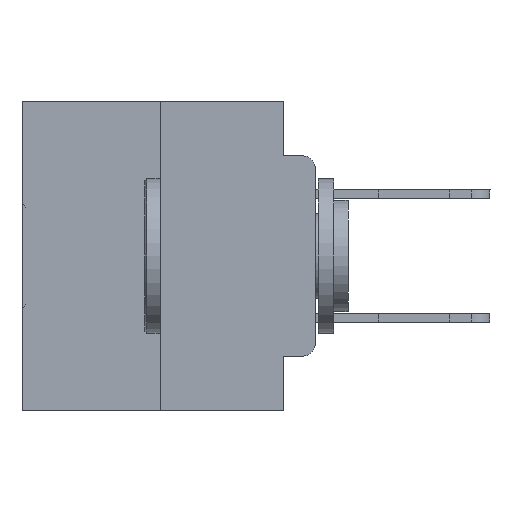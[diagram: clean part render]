
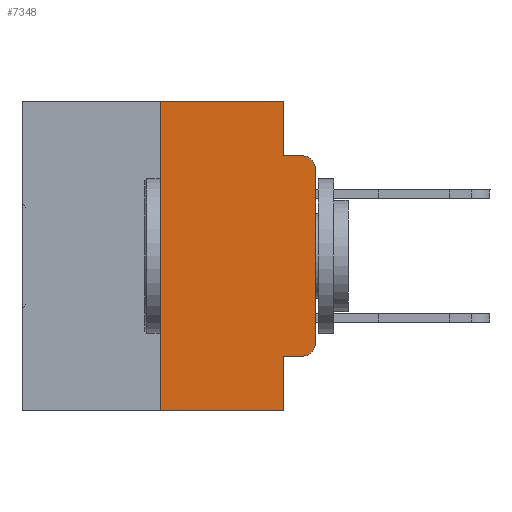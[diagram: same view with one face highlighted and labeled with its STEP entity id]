
A CAD part, left-side view. The second image highlights one B-rep face of the part: STEP entity #7348.
In plain terms, the highlighted planar face has unit normal (-1, 0, 0).
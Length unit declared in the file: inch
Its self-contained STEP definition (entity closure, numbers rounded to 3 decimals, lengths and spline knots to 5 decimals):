
#79 = DIRECTION ( 'NONE',  ( 0., 0., -1. ) ) ;
#104 = VERTEX_POINT ( 'NONE', #13565 ) ;
#146 = LINE ( 'NONE', #10324, #1235 ) ;
#973 = EDGE_LOOP ( 'NONE', ( #5817, #30918, #27660, #21546, #10218, #32575, #21661, #21333, #32468, #3909 ) ) ;
#1235 = VECTOR ( 'NONE', #27585, 39.37008 ) ;
#1272 = VECTOR ( 'NONE', #16689, 39.37008 ) ;
#1779 = CARTESIAN_POINT ( 'NONE',  ( 0., 0.473, 0. ) ) ;
#1830 = VERTEX_POINT ( 'NONE', #13114 ) ;
#3909 = ORIENTED_EDGE ( 'NONE', *, *, #12472, .T. ) ;
#4030 = VECTOR ( 'NONE', #15948, 39.37008 ) ;
#4287 = FACE_OUTER_BOUND ( 'NONE', #973, .T. ) ;
#4289 = VERTEX_POINT ( 'NONE', #6188 ) ;
#4841 = CARTESIAN_POINT ( 'NONE',  ( 0., 0.051, -0.5 ) ) ;
#4871 = VECTOR ( 'NONE', #7489, 39.37008 ) ;
#5817 = ORIENTED_EDGE ( 'NONE', *, *, #18081, .T. ) ;
#5888 = AXIS2_PLACEMENT_3D ( 'NONE', #1779, #7111, #12622 ) ;
#6101 = CIRCLE ( 'NONE', #8220, 0.02 ) ;
#6188 = CARTESIAN_POINT ( 'NONE',  ( 0., 0.051, -0.4115 ) ) ;
#6401 = CARTESIAN_POINT ( 'NONE',  ( 0., 0.25, 0. ) ) ;
#6491 = CARTESIAN_POINT ( 'NONE',  ( 0., 0.473, 0. ) ) ;
#7111 = DIRECTION ( 'NONE',  ( 1., 0., 0. ) ) ;
#7268 = DIRECTION ( 'NONE',  ( 0., 0., -1. ) ) ;
#7325 = VERTEX_POINT ( 'NONE', #32881 ) ;
#7348 = ADVANCED_FACE ( 'NONE', ( #4287 ), #27689, .F. ) ;
#7489 = DIRECTION ( 'NONE',  ( 0., 0., 1. ) ) ;
#8084 = LINE ( 'NONE', #23482, #4030 ) ;
#8220 = AXIS2_PLACEMENT_3D ( 'NONE', #19457, #29670, #29835 ) ;
#10218 = ORIENTED_EDGE ( 'NONE', *, *, #25123, .F. ) ;
#10324 = CARTESIAN_POINT ( 'NONE',  ( 0., 0., 0. ) ) ;
#10614 = EDGE_CURVE ( 'NONE', #7325, #20642, #23380, .T. ) ;
#11240 = CARTESIAN_POINT ( 'NONE',  ( 0., 0.02, -0.4115 ) ) ;
#11770 = DIRECTION ( 'NONE',  ( -1., 0., 0. ) ) ;
#12216 = VERTEX_POINT ( 'NONE', #4841 ) ;
#12270 = DIRECTION ( 'NONE',  ( 0., -1., 0. ) ) ;
#12472 = EDGE_CURVE ( 'NONE', #27366, #30332, #25313, .T. ) ;
#12622 = DIRECTION ( 'NONE',  ( 0., 0., -1. ) ) ;
#12770 = LINE ( 'NONE', #22987, #32877 ) ;
#13114 = CARTESIAN_POINT ( 'NONE',  ( 0., 0.02, -0.0885 ) ) ;
#13565 = CARTESIAN_POINT ( 'NONE',  ( 0., 0.051, -0.0885 ) ) ;
#13843 = LINE ( 'NONE', #6491, #1272 ) ;
#14895 = VERTEX_POINT ( 'NONE', #29708 ) ;
#15690 = DIRECTION ( 'NONE',  ( 0., 0., -1. ) ) ;
#15948 = DIRECTION ( 'NONE',  ( 0., -1., 0. ) ) ;
#16689 = DIRECTION ( 'NONE',  ( 0., -1., 0. ) ) ;
#17409 = EDGE_CURVE ( 'NONE', #31942, #104, #20246, .T. ) ;
#17559 = CARTESIAN_POINT ( 'NONE',  ( 0., 0.051, 0. ) ) ;
#18081 = EDGE_CURVE ( 'NONE', #30332, #14895, #146, .T. ) ;
#18428 = VECTOR ( 'NONE', #29647, 39.37008 ) ;
#18821 = VECTOR ( 'NONE', #15690, 39.37008 ) ;
#19030 = CARTESIAN_POINT ( 'NONE',  ( 0., 0.051, 0. ) ) ;
#19457 = CARTESIAN_POINT ( 'NONE',  ( 0., 0.02, -0.1085 ) ) ;
#19657 = CARTESIAN_POINT ( 'NONE',  ( 0., 0.051, -0.4115 ) ) ;
#19978 = CARTESIAN_POINT ( 'NONE',  ( 0., 0.02, -0.3915 ) ) ;
#20221 = CARTESIAN_POINT ( 'NONE',  ( 0., 0.25, 0. ) ) ;
#20246 = LINE ( 'NONE', #17559, #18821 ) ;
#20357 = EDGE_CURVE ( 'NONE', #4289, #12216, #12770, .T. ) ;
#20642 = VERTEX_POINT ( 'NONE', #6401 ) ;
#21333 = ORIENTED_EDGE ( 'NONE', *, *, #20357, .F. ) ;
#21546 = ORIENTED_EDGE ( 'NONE', *, *, #17409, .F. ) ;
#21661 = ORIENTED_EDGE ( 'NONE', *, *, #31012, .T. ) ;
#21738 = VECTOR ( 'NONE', #12270, 39.37008 ) ;
#21763 = EDGE_CURVE ( 'NONE', #104, #1830, #8084, .T. ) ;
#22656 = LINE ( 'NONE', #19657, #21738 ) ;
#22987 = CARTESIAN_POINT ( 'NONE',  ( 0., 0.051, 0. ) ) ;
#23380 = LINE ( 'NONE', #20221, #4871 ) ;
#23482 = CARTESIAN_POINT ( 'NONE',  ( 0., 0.051, -0.0885 ) ) ;
#24193 = EDGE_CURVE ( 'NONE', #14895, #1830, #6101, .T. ) ;
#24451 = CARTESIAN_POINT ( 'NONE',  ( 0., 0.473, -0.5 ) ) ;
#25123 = EDGE_CURVE ( 'NONE', #20642, #31942, #13843, .T. ) ;
#25313 = CIRCLE ( 'NONE', #28505, 0.02 ) ;
#27366 = VERTEX_POINT ( 'NONE', #11240 ) ;
#27585 = DIRECTION ( 'NONE',  ( 0., 0., 1. ) ) ;
#27660 = ORIENTED_EDGE ( 'NONE', *, *, #21763, .F. ) ;
#27689 = PLANE ( 'NONE',  #5888 ) ;
#28344 = CARTESIAN_POINT ( 'NONE',  ( 0., 0., -0.3915 ) ) ;
#28505 = AXIS2_PLACEMENT_3D ( 'NONE', #19978, #11770, #7268 ) ;
#29647 = DIRECTION ( 'NONE',  ( 0., -1., 0. ) ) ;
#29670 = DIRECTION ( 'NONE',  ( -1., 0., 0. ) ) ;
#29708 = CARTESIAN_POINT ( 'NONE',  ( 0., 0., -0.1085 ) ) ;
#29809 = LINE ( 'NONE', #24451, #18428 ) ;
#29835 = DIRECTION ( 'NONE',  ( 0., 0., -1. ) ) ;
#30332 = VERTEX_POINT ( 'NONE', #28344 ) ;
#30918 = ORIENTED_EDGE ( 'NONE', *, *, #24193, .T. ) ;
#31012 = EDGE_CURVE ( 'NONE', #7325, #12216, #29809, .T. ) ;
#31942 = VERTEX_POINT ( 'NONE', #19030 ) ;
#32468 = ORIENTED_EDGE ( 'NONE', *, *, #32698, .T. ) ;
#32575 = ORIENTED_EDGE ( 'NONE', *, *, #10614, .F. ) ;
#32698 = EDGE_CURVE ( 'NONE', #4289, #27366, #22656, .T. ) ;
#32877 = VECTOR ( 'NONE', #79, 39.37008 ) ;
#32881 = CARTESIAN_POINT ( 'NONE',  ( 0., 0.25, -0.5 ) ) ;
